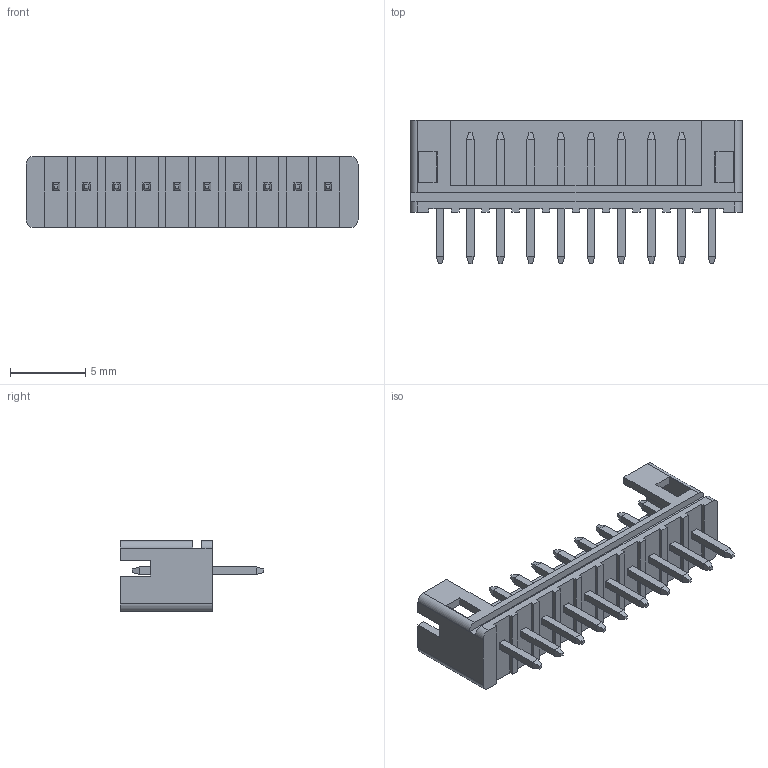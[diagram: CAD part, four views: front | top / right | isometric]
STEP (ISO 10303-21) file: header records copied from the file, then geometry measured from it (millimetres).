
FILE_DESCRIPTION (( 'STEP AP203' ), '1' );
FILE_NAME ('140-510-415-101.STEP', '2020-09-25T11:17:45', ( '' ), ( '' ), 'SwSTEP 2.0', 'SolidWorks 2020', '' );
FILE_SCHEMA (( 'CONFIG_CONTROL_DESIGN' ));
Length unit declared in the file: millimetre
Products named in the file (3): V LI Contact_Str; V LI Housing_510; 140-510-415-101
Assembly tree (11 placements, depth 2):
  140-510-415-101
    V LI Housing_510
    V LI Contact_Str  x10
Bounding box: 22 x 9.5 x 4.7 mm (x, y, z)
Volume: 232.4 mm3; surface area: 849.8 mm2
Topology: 11 solids, 11 shells, 260 faces, 636 edges, 396 vertices
Faces by surface type: plane 254, cylinder 6
Entity records: 4925 total; most frequent: CARTESIAN_POINT 784, ORIENTED_EDGE 768, DIRECTION 692, EDGE_CURVE 384, VECTOR 372, LINE 372, VERTEX_POINT 252, AXIS2_PLACEMENT_3D 160
